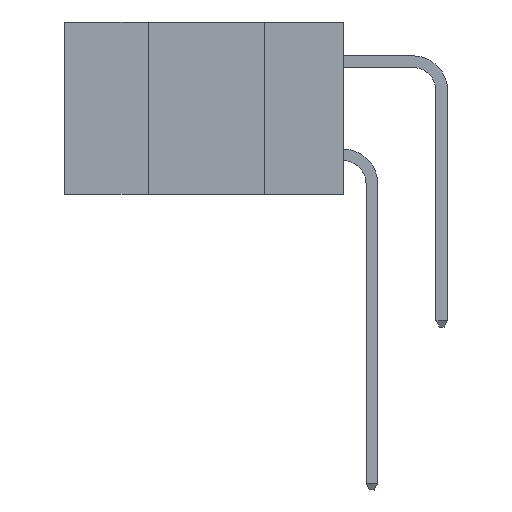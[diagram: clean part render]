
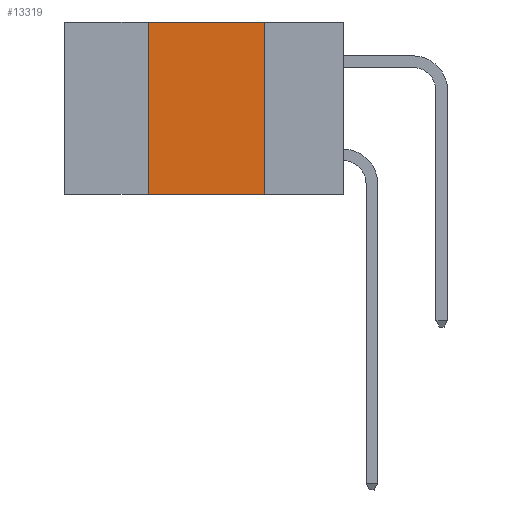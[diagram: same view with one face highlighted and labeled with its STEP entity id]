
A CAD part, left-side view. The second image highlights one B-rep face of the part: STEP entity #13319.
In plain terms, the highlighted planar face has unit normal (-1, 0, 0).
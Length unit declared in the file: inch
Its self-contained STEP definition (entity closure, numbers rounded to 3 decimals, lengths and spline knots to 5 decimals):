
#1232 = LINE ( 'NONE', #16227, #28619 ) ;
#2399 = AXIS2_PLACEMENT_3D ( 'NONE', #17560, #20261, #28183 ) ;
#3256 = ORIENTED_EDGE ( 'NONE', *, *, #20679, .F. ) ;
#3741 = VERTEX_POINT ( 'NONE', #5758 ) ;
#4309 = CARTESIAN_POINT ( 'NONE',  ( 0., 0.17, -0.37 ) ) ;
#5374 = ORIENTED_EDGE ( 'NONE', *, *, #19007, .T. ) ;
#5758 = CARTESIAN_POINT ( 'NONE',  ( 0., 0.17, 0. ) ) ;
#6439 = VERTEX_POINT ( 'NONE', #30268 ) ;
#6642 = VERTEX_POINT ( 'NONE', #26580 ) ;
#9733 = CARTESIAN_POINT ( 'NONE',  ( 0., 0.42, 0. ) ) ;
#10487 = DIRECTION ( 'NONE',  ( 0., -1., 0. ) ) ;
#10852 = FACE_OUTER_BOUND ( 'NONE', #14714, .T. ) ;
#12398 = DIRECTION ( 'NONE',  ( 0., -1., 0. ) ) ;
#12969 = ORIENTED_EDGE ( 'NONE', *, *, #22544, .F. ) ;
#13319 = ADVANCED_FACE ( 'NONE', ( #10852 ), #33214, .F. ) ;
#13818 = LINE ( 'NONE', #33174, #17486 ) ;
#14714 = EDGE_LOOP ( 'NONE', ( #21399, #3256, #12969, #5374 ) ) ;
#15992 = VECTOR ( 'NONE', #10487, 39.37008 ) ;
#16227 = CARTESIAN_POINT ( 'NONE',  ( 0., 0.17, 0. ) ) ;
#17486 = VECTOR ( 'NONE', #12398, 39.37008 ) ;
#17560 = CARTESIAN_POINT ( 'NONE',  ( 0., 0.6, 0. ) ) ;
#19007 = EDGE_CURVE ( 'NONE', #6439, #26105, #22983, .T. ) ;
#19454 = EDGE_CURVE ( 'NONE', #3741, #26105, #1232, .T. ) ;
#20261 = DIRECTION ( 'NONE',  ( 1., 0., 0. ) ) ;
#20679 = EDGE_CURVE ( 'NONE', #6642, #3741, #13818, .T. ) ;
#21399 = ORIENTED_EDGE ( 'NONE', *, *, #19454, .F. ) ;
#22544 = EDGE_CURVE ( 'NONE', #6439, #6642, #23128, .T. ) ;
#22919 = DIRECTION ( 'NONE',  ( 0., 0., 1. ) ) ;
#22983 = LINE ( 'NONE', #26123, #15992 ) ;
#23128 = LINE ( 'NONE', #9733, #28822 ) ;
#24049 = DIRECTION ( 'NONE',  ( 0., 0., -1. ) ) ;
#26105 = VERTEX_POINT ( 'NONE', #4309 ) ;
#26123 = CARTESIAN_POINT ( 'NONE',  ( 0., 0.6, -0.37 ) ) ;
#26580 = CARTESIAN_POINT ( 'NONE',  ( 0., 0.42, 0. ) ) ;
#28183 = DIRECTION ( 'NONE',  ( 0., 0., -1. ) ) ;
#28619 = VECTOR ( 'NONE', #24049, 39.37008 ) ;
#28822 = VECTOR ( 'NONE', #22919, 39.37008 ) ;
#30268 = CARTESIAN_POINT ( 'NONE',  ( 0., 0.42, -0.37 ) ) ;
#33174 = CARTESIAN_POINT ( 'NONE',  ( 0., 0.6, 0. ) ) ;
#33214 = PLANE ( 'NONE',  #2399 ) ;
